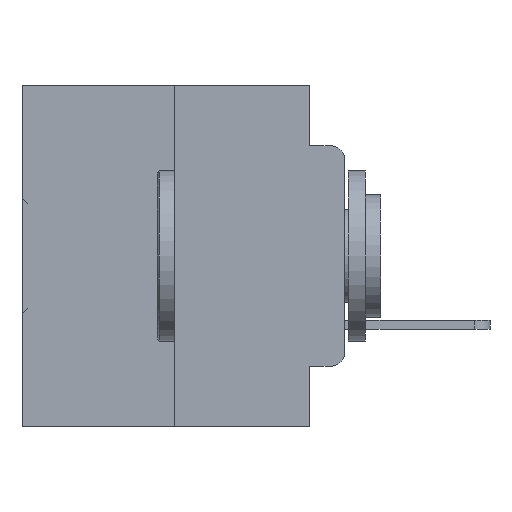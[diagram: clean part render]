
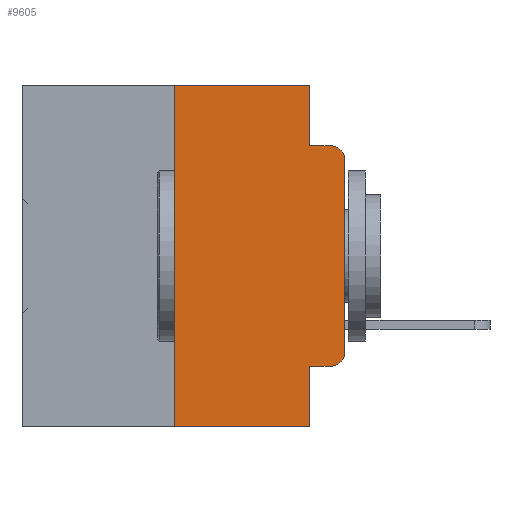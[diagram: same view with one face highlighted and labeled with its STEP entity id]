
A CAD part, left-side view. The second image highlights one B-rep face of the part: STEP entity #9605.
In plain terms, the highlighted planar face has unit normal (-1, 0, 0).
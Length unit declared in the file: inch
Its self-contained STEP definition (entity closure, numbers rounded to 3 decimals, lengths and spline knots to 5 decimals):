
#79 = VERTEX_POINT ( 'NONE', #453 ) ;
#431 = FACE_OUTER_BOUND ( 'NONE', #10400, .T. ) ;
#453 = CARTESIAN_POINT ( 'NONE',  ( 0., 0.25, -0.5 ) ) ;
#1073 = EDGE_CURVE ( 'NONE', #79, #6380, #3905, .T. ) ;
#1845 = CARTESIAN_POINT ( 'NONE',  ( 0., 0.051, -0.4115 ) ) ;
#2417 = ORIENTED_EDGE ( 'NONE', *, *, #29790, .T. ) ;
#2875 = DIRECTION ( 'NONE',  ( 0., -1., 0. ) ) ;
#2916 = VECTOR ( 'NONE', #7857, 39.37008 ) ;
#3049 = EDGE_CURVE ( 'NONE', #6142, #6836, #4721, .T. ) ;
#3905 = LINE ( 'NONE', #29088, #17242 ) ;
#3935 = CARTESIAN_POINT ( 'NONE',  ( 0., 0.051, -0.4115 ) ) ;
#4109 = CARTESIAN_POINT ( 'NONE',  ( 0., 0.473, -0.5 ) ) ;
#4233 = CIRCLE ( 'NONE', #31146, 0.02 ) ;
#4721 = LINE ( 'NONE', #21897, #2916 ) ;
#5979 = AXIS2_PLACEMENT_3D ( 'NONE', #24180, #7288, #26938 ) ;
#6142 = VERTEX_POINT ( 'NONE', #7958 ) ;
#6380 = VERTEX_POINT ( 'NONE', #34031 ) ;
#6836 = VERTEX_POINT ( 'NONE', #16706 ) ;
#6886 = ORIENTED_EDGE ( 'NONE', *, *, #19218, .F. ) ;
#7051 = PLANE ( 'NONE',  #25972 ) ;
#7074 = CARTESIAN_POINT ( 'NONE',  ( 0., 0.02, -0.4115 ) ) ;
#7282 = VERTEX_POINT ( 'NONE', #1845 ) ;
#7288 = DIRECTION ( 'NONE',  ( -1., 0., 0. ) ) ;
#7326 = CARTESIAN_POINT ( 'NONE',  ( 0., 0.02, -0.0885 ) ) ;
#7857 = DIRECTION ( 'NONE',  ( 0., 0., 1. ) ) ;
#7958 = CARTESIAN_POINT ( 'NONE',  ( 0., 0., -0.3915 ) ) ;
#8688 = ORIENTED_EDGE ( 'NONE', *, *, #19917, .F. ) ;
#9605 = ADVANCED_FACE ( 'NONE', ( #431 ), #7051, .F. ) ;
#9713 = LINE ( 'NONE', #4109, #15433 ) ;
#9902 = CARTESIAN_POINT ( 'NONE',  ( 0., 0.473, 0. ) ) ;
#10400 = EDGE_LOOP ( 'NONE', ( #29197, #12219, #6886, #8688, #10464, #28833, #2417, #20165, #17120, #33473 ) ) ;
#10464 = ORIENTED_EDGE ( 'NONE', *, *, #32110, .F. ) ;
#12219 = ORIENTED_EDGE ( 'NONE', *, *, #24145, .T. ) ;
#12750 = DIRECTION ( 'NONE',  ( 0., 0., -1. ) ) ;
#12804 = DIRECTION ( 'NONE',  ( 0., 0., -1. ) ) ;
#13402 = VERTEX_POINT ( 'NONE', #7326 ) ;
#13428 = CARTESIAN_POINT ( 'NONE',  ( 0., 0.051, 0. ) ) ;
#13585 = LINE ( 'NONE', #13428, #20113 ) ;
#13612 = VECTOR ( 'NONE', #21086, 39.37008 ) ;
#14116 = DIRECTION ( 'NONE',  ( -1., 0., 0. ) ) ;
#14652 = VERTEX_POINT ( 'NONE', #33650 ) ;
#14889 = LINE ( 'NONE', #29395, #35955 ) ;
#15433 = VECTOR ( 'NONE', #29402, 39.37008 ) ;
#15438 = CARTESIAN_POINT ( 'NONE',  ( 0., 0.473, 0. ) ) ;
#16706 = CARTESIAN_POINT ( 'NONE',  ( 0., 0., -0.1085 ) ) ;
#17120 = ORIENTED_EDGE ( 'NONE', *, *, #25957, .T. ) ;
#17242 = VECTOR ( 'NONE', #23371, 39.37008 ) ;
#19211 = VERTEX_POINT ( 'NONE', #36080 ) ;
#19218 = EDGE_CURVE ( 'NONE', #35907, #13402, #31816, .T. ) ;
#19696 = VECTOR ( 'NONE', #29246, 39.37008 ) ;
#19917 = EDGE_CURVE ( 'NONE', #14652, #35907, #14889, .T. ) ;
#20113 = VECTOR ( 'NONE', #35393, 39.37008 ) ;
#20165 = ORIENTED_EDGE ( 'NONE', *, *, #33187, .F. ) ;
#20994 = LINE ( 'NONE', #15438, #13612 ) ;
#21086 = DIRECTION ( 'NONE',  ( 0., -1., 0. ) ) ;
#21897 = CARTESIAN_POINT ( 'NONE',  ( 0., 0., 0. ) ) ;
#22653 = CARTESIAN_POINT ( 'NONE',  ( 0., 0.051, -0.0885 ) ) ;
#23371 = DIRECTION ( 'NONE',  ( 0., 0., 1. ) ) ;
#23741 = VECTOR ( 'NONE', #2875, 39.37008 ) ;
#24145 = EDGE_CURVE ( 'NONE', #6836, #13402, #4233, .T. ) ;
#24180 = CARTESIAN_POINT ( 'NONE',  ( 0., 0.02, -0.3915 ) ) ;
#25292 = CIRCLE ( 'NONE', #5979, 0.02 ) ;
#25957 = EDGE_CURVE ( 'NONE', #7282, #34827, #27952, .T. ) ;
#25972 = AXIS2_PLACEMENT_3D ( 'NONE', #9902, #29444, #12804 ) ;
#26938 = DIRECTION ( 'NONE',  ( 0., 0., -1. ) ) ;
#27321 = EDGE_CURVE ( 'NONE', #34827, #6142, #25292, .T. ) ;
#27952 = LINE ( 'NONE', #3935, #19696 ) ;
#28833 = ORIENTED_EDGE ( 'NONE', *, *, #1073, .F. ) ;
#29088 = CARTESIAN_POINT ( 'NONE',  ( 0., 0.25, 0. ) ) ;
#29197 = ORIENTED_EDGE ( 'NONE', *, *, #3049, .T. ) ;
#29246 = DIRECTION ( 'NONE',  ( 0., -1., 0. ) ) ;
#29395 = CARTESIAN_POINT ( 'NONE',  ( 0., 0.051, 0. ) ) ;
#29402 = DIRECTION ( 'NONE',  ( 0., -1., 0. ) ) ;
#29444 = DIRECTION ( 'NONE',  ( 1., 0., 0. ) ) ;
#29790 = EDGE_CURVE ( 'NONE', #79, #19211, #9713, .T. ) ;
#30590 = CARTESIAN_POINT ( 'NONE',  ( 0., 0.051, -0.0885 ) ) ;
#30677 = CARTESIAN_POINT ( 'NONE',  ( 0., 0.02, -0.1085 ) ) ;
#31146 = AXIS2_PLACEMENT_3D ( 'NONE', #30677, #14116, #33378 ) ;
#31816 = LINE ( 'NONE', #22653, #23741 ) ;
#32110 = EDGE_CURVE ( 'NONE', #6380, #14652, #20994, .T. ) ;
#33187 = EDGE_CURVE ( 'NONE', #7282, #19211, #13585, .T. ) ;
#33378 = DIRECTION ( 'NONE',  ( 0., 0., -1. ) ) ;
#33473 = ORIENTED_EDGE ( 'NONE', *, *, #27321, .T. ) ;
#33650 = CARTESIAN_POINT ( 'NONE',  ( 0., 0.051, 0. ) ) ;
#34031 = CARTESIAN_POINT ( 'NONE',  ( 0., 0.25, 0. ) ) ;
#34827 = VERTEX_POINT ( 'NONE', #7074 ) ;
#35393 = DIRECTION ( 'NONE',  ( 0., 0., -1. ) ) ;
#35907 = VERTEX_POINT ( 'NONE', #30590 ) ;
#35955 = VECTOR ( 'NONE', #12750, 39.37008 ) ;
#36080 = CARTESIAN_POINT ( 'NONE',  ( 0., 0.051, -0.5 ) ) ;
